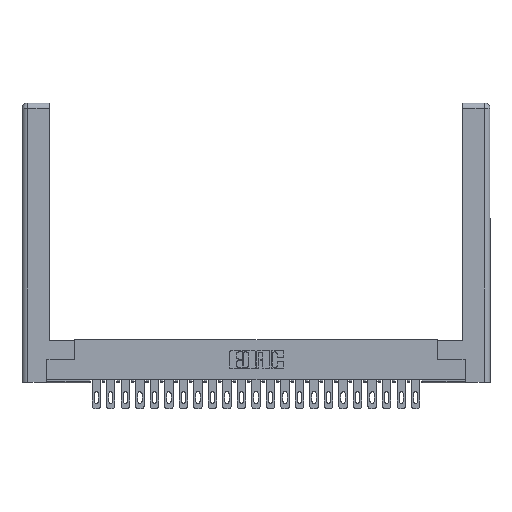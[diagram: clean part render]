
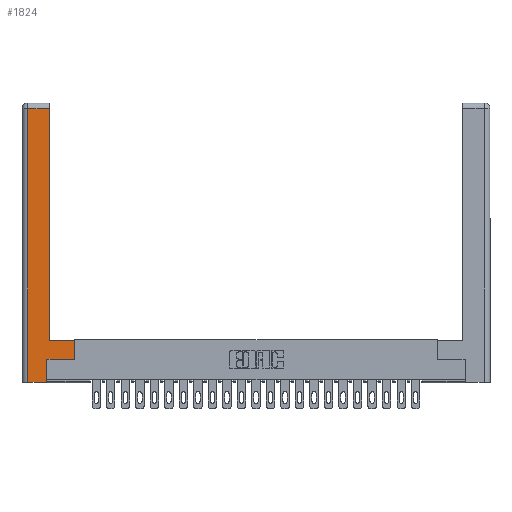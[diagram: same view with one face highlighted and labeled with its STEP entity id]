
A CAD part, top view. The second image highlights one B-rep face of the part: STEP entity #1824.
In plain terms, the highlighted planar face has unit normal (0, 0, 1).
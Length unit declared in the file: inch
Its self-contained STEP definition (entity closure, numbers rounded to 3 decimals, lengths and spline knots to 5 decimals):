
#190 = LINE ( 'NONE', #20930, #10996 ) ;
#354 = CARTESIAN_POINT ( 'NONE',  ( 0.295, 0.45, 0. ) ) ;
#748 = CARTESIAN_POINT ( 'NONE',  ( 0.565, 0.245, 0. ) ) ;
#1302 = CARTESIAN_POINT ( 'NONE',  ( 0.0615, 0., 0. ) ) ;
#1706 = ORIENTED_EDGE ( 'NONE', *, *, #5757, .T. ) ;
#1814 = LINE ( 'NONE', #354, #10487 ) ;
#1824 = ADVANCED_FACE ( 'NONE', ( #22823 ), #9108, .F. ) ;
#2454 = LINE ( 'NONE', #13033, #7107 ) ;
#2547 = DIRECTION ( 'NONE',  ( -1., 0., 0. ) ) ;
#2665 = EDGE_CURVE ( 'NONE', #17587, #4686, #1814, .T. ) ;
#2854 = CARTESIAN_POINT ( 'NONE',  ( 0.295, 3., 0. ) ) ;
#3831 = ORIENTED_EDGE ( 'NONE', *, *, #10082, .T. ) ;
#4686 = VERTEX_POINT ( 'NONE', #19808 ) ;
#5738 = ORIENTED_EDGE ( 'NONE', *, *, #2665, .T. ) ;
#5757 = EDGE_CURVE ( 'NONE', #10279, #25624, #15029, .T. ) ;
#6244 = CARTESIAN_POINT ( 'NONE',  ( 0.0615, 0., 0. ) ) ;
#6302 = VERTEX_POINT ( 'NONE', #1302 ) ;
#6698 = DIRECTION ( 'NONE',  ( 0., 1., 0. ) ) ;
#6889 = ORIENTED_EDGE ( 'NONE', *, *, #29895, .T. ) ;
#7107 = VECTOR ( 'NONE', #24727, 39.37008 ) ;
#7141 = EDGE_CURVE ( 'NONE', #4686, #10279, #22640, .T. ) ;
#7974 = VERTEX_POINT ( 'NONE', #23611 ) ;
#8931 = CARTESIAN_POINT ( 'NONE',  ( 0.565, 0.45, 0. ) ) ;
#9108 = PLANE ( 'NONE',  #14443 ) ;
#9191 = CARTESIAN_POINT ( 'NONE',  ( 0.0615, 2.94, 0. ) ) ;
#9239 = ORIENTED_EDGE ( 'NONE', *, *, #20185, .T. ) ;
#9407 = DIRECTION ( 'NONE',  ( -1., 0., 0. ) ) ;
#10082 = EDGE_CURVE ( 'NONE', #25624, #6302, #17806, .T. ) ;
#10279 = VERTEX_POINT ( 'NONE', #18505 ) ;
#10487 = VECTOR ( 'NONE', #9407, 39.37008 ) ;
#10996 = VECTOR ( 'NONE', #25411, 39.37008 ) ;
#13033 = CARTESIAN_POINT ( 'NONE',  ( 0.265, 0., 0. ) ) ;
#14443 = AXIS2_PLACEMENT_3D ( 'NONE', #22939, #27782, #2547 ) ;
#14614 = ORIENTED_EDGE ( 'NONE', *, *, #28885, .T. ) ;
#14770 = CARTESIAN_POINT ( 'NONE',  ( 0.265, 0.245, 0. ) ) ;
#15029 = LINE ( 'NONE', #22834, #20067 ) ;
#15163 = VECTOR ( 'NONE', #29051, 39.37008 ) ;
#17162 = CARTESIAN_POINT ( 'NONE',  ( 0.565, 0.245, 0. ) ) ;
#17587 = VERTEX_POINT ( 'NONE', #8931 ) ;
#17806 = LINE ( 'NONE', #6244, #22068 ) ;
#18322 = DIRECTION ( 'NONE',  ( -1., 0., 0. ) ) ;
#18505 = CARTESIAN_POINT ( 'NONE',  ( 0.295, 2.94, 0. ) ) ;
#19243 = VECTOR ( 'NONE', #6698, 39.37008 ) ;
#19808 = CARTESIAN_POINT ( 'NONE',  ( 0.295, 0.45, 0. ) ) ;
#19921 = EDGE_CURVE ( 'NONE', #29503, #17587, #26086, .T. ) ;
#20067 = VECTOR ( 'NONE', #18322, 39.37008 ) ;
#20185 = EDGE_CURVE ( 'NONE', #7974, #29721, #190, .T. ) ;
#20532 = CARTESIAN_POINT ( 'NONE',  ( 0.565, 0.45, 0. ) ) ;
#20930 = CARTESIAN_POINT ( 'NONE',  ( 0.265, 0.245, 0. ) ) ;
#21435 = ORIENTED_EDGE ( 'NONE', *, *, #7141, .T. ) ;
#22068 = VECTOR ( 'NONE', #29089, 39.37008 ) ;
#22640 = LINE ( 'NONE', #2854, #24429 ) ;
#22749 = LINE ( 'NONE', #17162, #15163 ) ;
#22823 = FACE_OUTER_BOUND ( 'NONE', #23544, .T. ) ;
#22834 = CARTESIAN_POINT ( 'NONE',  ( 0.0615, 2.94, 0. ) ) ;
#22939 = CARTESIAN_POINT ( 'NONE',  ( 0., 0., 0. ) ) ;
#23544 = EDGE_LOOP ( 'NONE', ( #21435, #1706, #3831, #6889, #9239, #14614, #27161, #5738 ) ) ;
#23611 = CARTESIAN_POINT ( 'NONE',  ( 0.265, 0., 0. ) ) ;
#24429 = VECTOR ( 'NONE', #25953, 39.37008 ) ;
#24727 = DIRECTION ( 'NONE',  ( 1., 0., 0. ) ) ;
#25411 = DIRECTION ( 'NONE',  ( 0., 1., 0. ) ) ;
#25624 = VERTEX_POINT ( 'NONE', #9191 ) ;
#25953 = DIRECTION ( 'NONE',  ( 0., 1., 0. ) ) ;
#26086 = LINE ( 'NONE', #20532, #19243 ) ;
#27161 = ORIENTED_EDGE ( 'NONE', *, *, #19921, .T. ) ;
#27782 = DIRECTION ( 'NONE',  ( 0., 0., -1. ) ) ;
#28885 = EDGE_CURVE ( 'NONE', #29721, #29503, #22749, .T. ) ;
#29051 = DIRECTION ( 'NONE',  ( 1., 0., 0. ) ) ;
#29089 = DIRECTION ( 'NONE',  ( 0., -1., 0. ) ) ;
#29503 = VERTEX_POINT ( 'NONE', #748 ) ;
#29721 = VERTEX_POINT ( 'NONE', #14770 ) ;
#29895 = EDGE_CURVE ( 'NONE', #6302, #7974, #2454, .T. ) ;
